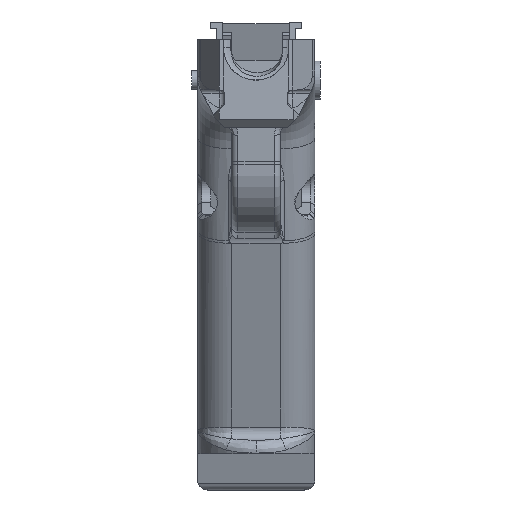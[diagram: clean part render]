
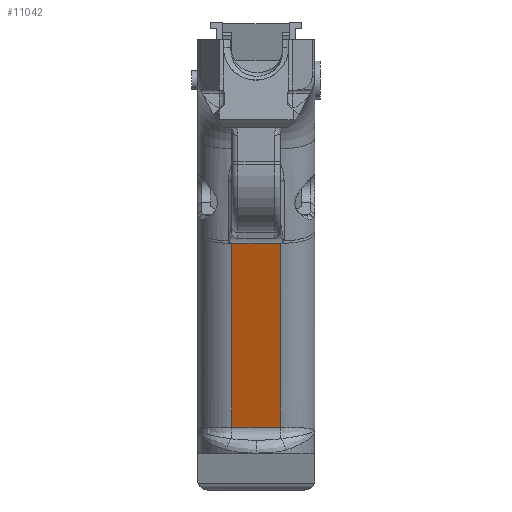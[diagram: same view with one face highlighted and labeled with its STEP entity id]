
A CAD part, front view. The second image highlights one B-rep face of the part: STEP entity #11042.
In plain terms, the highlighted planar face has unit normal (0, -0.947, -0.322).
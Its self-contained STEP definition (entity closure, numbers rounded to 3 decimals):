
#1198=FACE_OUTER_BOUND('',#1813,.T.);
#1813=EDGE_LOOP('',(#9330,#9331,#9332,#9333));
#2346=LINE('',#15660,#3503);
#3016=LINE('',#18810,#4173);
#3017=LINE('',#18830,#4174);
#3018=LINE('',#18831,#4175);
#3503=VECTOR('',#12832,10.);
#4173=VECTOR('',#14282,10.);
#4174=VECTOR('',#14287,10.);
#4175=VECTOR('',#14288,10.);
#4572=VERTEX_POINT('',#15657);
#4573=VERTEX_POINT('',#15659);
#5197=VERTEX_POINT('',#18802);
#5198=VERTEX_POINT('',#18809);
#5757=EDGE_CURVE('',#4572,#4573,#2346,.T.);
#6664=EDGE_CURVE('',#5197,#5198,#3016,.T.);
#6668=EDGE_CURVE('',#5198,#4572,#3017,.T.);
#6669=EDGE_CURVE('',#4573,#5197,#3018,.T.);
#9330=ORIENTED_EDGE('',*,*,#6668,.F.);
#9331=ORIENTED_EDGE('',*,*,#6664,.F.);
#9332=ORIENTED_EDGE('',*,*,#6669,.F.);
#9333=ORIENTED_EDGE('',*,*,#5757,.F.);
#10570=PLANE('',#11889);
#11042=ADVANCED_FACE('',(#1198),#10570,.T.);
#11889=AXIS2_PLACEMENT_3D('',#18829,#14285,#14286);
#12832=DIRECTION('',(0.,-0.322,0.947));
#14282=DIRECTION('',(0.,0.322,-0.947));
#14285=DIRECTION('center_axis',(0.,-0.947,-0.322));
#14286=DIRECTION('ref_axis',(0.,0.322,-0.947));
#14287=DIRECTION('',(-1.,0.,0.));
#14288=DIRECTION('',(1.,0.,0.));
#15657=CARTESIAN_POINT('',(-14.218,-62.644,-85.79));
#15659=CARTESIAN_POINT('',(-14.218,-78.109,-40.345));
#15660=CARTESIAN_POINT('',(-14.218,-83.303,-25.083));
#18802=CARTESIAN_POINT('',(-2.118,-78.109,-40.345));
#18809=CARTESIAN_POINT('',(-2.118,-62.644,-85.79));
#18810=CARTESIAN_POINT('',(-2.118,-83.303,-25.083));
#18829=CARTESIAN_POINT('Origin',(-22.668,-78.109,-40.345));
#18830=CARTESIAN_POINT('',(-15.418,-62.644,-85.79));
#18831=CARTESIAN_POINT('',(0.,-78.109,-40.345));
